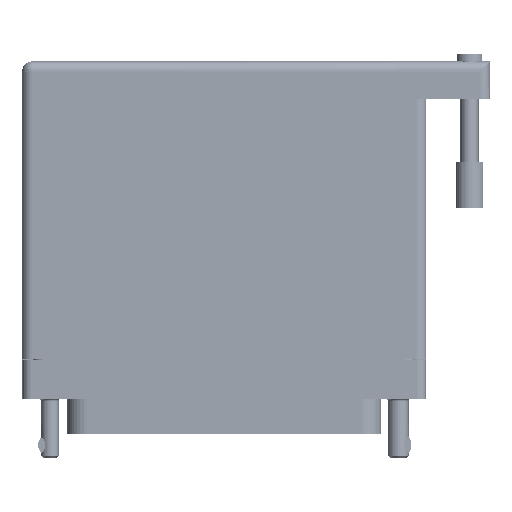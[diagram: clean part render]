
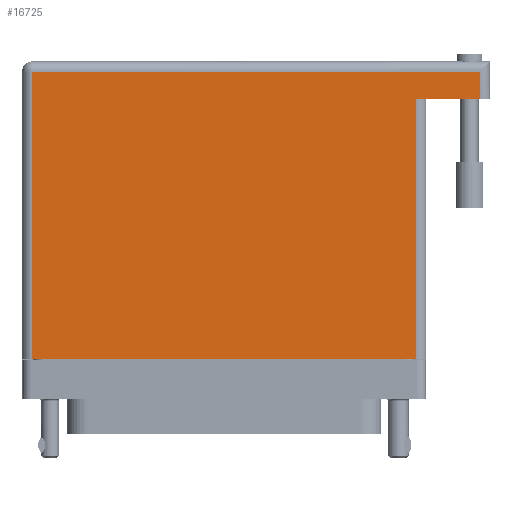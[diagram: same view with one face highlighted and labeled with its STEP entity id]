
A CAD part, front view. The second image highlights one B-rep face of the part: STEP entity #16725.
In plain terms, the highlighted face is planar.
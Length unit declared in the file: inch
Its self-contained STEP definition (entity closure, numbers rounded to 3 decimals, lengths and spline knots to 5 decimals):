
#7106 = CARTESIAN_POINT ( 'NONE',  ( 1.3075, 1.674, 0.765 ) ) ;
#8399 = FACE_OUTER_BOUND ( 'NONE', #89782, .T. ) ;
#11902 = EDGE_CURVE ( 'NONE', #28961, #15477, #28254, .T. ) ;
#14391 = LINE ( 'NONE', #83343, #28098 ) ;
#15064 = DIRECTION ( 'NONE',  ( 0., 1., 0. ) ) ;
#15477 = VERTEX_POINT ( 'NONE', #72043 ) ;
#16171 = LINE ( 'NONE', #92388, #55925 ) ;
#16725 = ADVANCED_FACE ( 'NONE', ( #8399 ), #64182, .F. ) ;
#16873 = AXIS2_PLACEMENT_3D ( 'NONE', #96081, #24678, #80153 ) ;
#17075 = ORIENTED_EDGE ( 'NONE', *, *, #28033, .T. ) ;
#20913 = ORIENTED_EDGE ( 'NONE', *, *, #89285, .T. ) ;
#22968 = CARTESIAN_POINT ( 'NONE',  ( 1.7425, 1.86, 0.765 ) ) ;
#23007 = DIRECTION ( 'NONE',  ( -1., 0., 0. ) ) ;
#23619 = CARTESIAN_POINT ( 'NONE',  ( -1.3775, -0.1, 0.765 ) ) ;
#24678 = DIRECTION ( 'NONE',  ( 0., 0., -1. ) ) ;
#24932 = VERTEX_POINT ( 'NONE', #22968 ) ;
#28033 = EDGE_CURVE ( 'NONE', #80862, #24932, #14391, .T. ) ;
#28098 = VECTOR ( 'NONE', #75982, 39.37008 ) ;
#28254 = LINE ( 'NONE', #23619, #31974 ) ;
#28961 = VERTEX_POINT ( 'NONE', #80933 ) ;
#31341 = ORIENTED_EDGE ( 'NONE', *, *, #11902, .T. ) ;
#31727 = CARTESIAN_POINT ( 'NONE',  ( 1.8125, 1.674, 0.765 ) ) ;
#31974 = VECTOR ( 'NONE', #48230, 39.37008 ) ;
#40630 = CARTESIAN_POINT ( 'NONE',  ( 1.7425, 1.674, 0.765 ) ) ;
#43455 = ORIENTED_EDGE ( 'NONE', *, *, #64967, .T. ) ;
#44103 = VECTOR ( 'NONE', #70143, 39.37008 ) ;
#44913 = DIRECTION ( 'NONE',  ( 0., -1., 0. ) ) ;
#45991 = ORIENTED_EDGE ( 'NONE', *, *, #87263, .F. ) ;
#48230 = DIRECTION ( 'NONE',  ( 1., 0., 0. ) ) ;
#54644 = LINE ( 'NONE', #7106, #83204 ) ;
#55925 = VECTOR ( 'NONE', #44913, 39.37008 ) ;
#56740 = VERTEX_POINT ( 'NONE', #73816 ) ;
#56875 = VECTOR ( 'NONE', #23007, 39.37008 ) ;
#57663 = LINE ( 'NONE', #93789, #44103 ) ;
#59220 = VERTEX_POINT ( 'NONE', #84432 ) ;
#62278 = ORIENTED_EDGE ( 'NONE', *, *, #71330, .T. ) ;
#64182 = PLANE ( 'NONE',  #16873 ) ;
#64967 = EDGE_CURVE ( 'NONE', #59220, #28961, #16171, .T. ) ;
#70143 = DIRECTION ( 'NONE',  ( -1., 0., 0. ) ) ;
#71330 = EDGE_CURVE ( 'NONE', #15477, #56740, #54644, .T. ) ;
#72043 = CARTESIAN_POINT ( 'NONE',  ( 1.3075, -0.1, 0.765 ) ) ;
#73816 = CARTESIAN_POINT ( 'NONE',  ( 1.3075, 1.674, 0.765 ) ) ;
#75982 = DIRECTION ( 'NONE',  ( 0., 1., 0. ) ) ;
#80153 = DIRECTION ( 'NONE',  ( -1., 0., 0. ) ) ;
#80862 = VERTEX_POINT ( 'NONE', #40630 ) ;
#80933 = CARTESIAN_POINT ( 'NONE',  ( -1.3075, -0.1, 0.765 ) ) ;
#83204 = VECTOR ( 'NONE', #15064, 39.37008 ) ;
#83343 = CARTESIAN_POINT ( 'NONE',  ( 1.7425, 1.93, 0.765 ) ) ;
#84432 = CARTESIAN_POINT ( 'NONE',  ( -1.3075, 1.86, 0.765 ) ) ;
#87263 = EDGE_CURVE ( 'NONE', #80862, #56740, #96568, .T. ) ;
#89285 = EDGE_CURVE ( 'NONE', #24932, #59220, #57663, .T. ) ;
#89782 = EDGE_LOOP ( 'NONE', ( #31341, #62278, #45991, #17075, #20913, #43455 ) ) ;
#92388 = CARTESIAN_POINT ( 'NONE',  ( -1.3075, -0.1, 0.765 ) ) ;
#93789 = CARTESIAN_POINT ( 'NONE',  ( -1.3775, 1.86, 0.765 ) ) ;
#96081 = CARTESIAN_POINT ( 'NONE',  ( -1.3775, 1.93, 0.765 ) ) ;
#96568 = LINE ( 'NONE', #31727, #56875 ) ;
